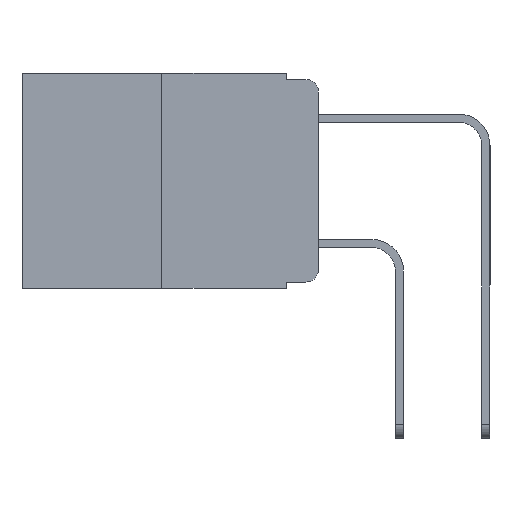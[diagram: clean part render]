
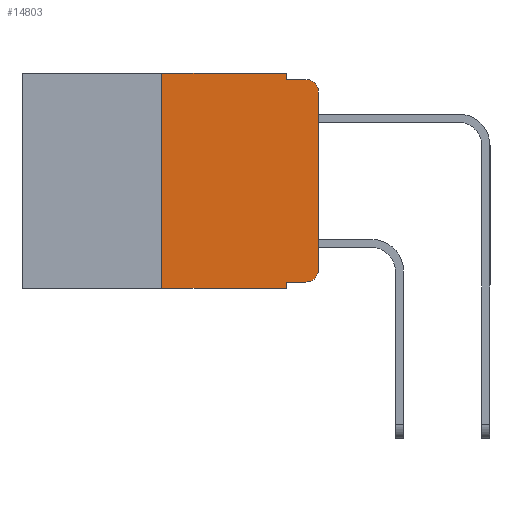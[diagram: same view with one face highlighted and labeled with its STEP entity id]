
A CAD part, left-side view. The second image highlights one B-rep face of the part: STEP entity #14803.
In plain terms, the highlighted planar face has unit normal (-1, 0, 0).
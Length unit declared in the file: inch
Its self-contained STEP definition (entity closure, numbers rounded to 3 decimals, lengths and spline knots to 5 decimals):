
#82 = VERTEX_POINT ( 'NONE', #9330 ) ;
#429 = VECTOR ( 'NONE', #21361, 39.37008 ) ;
#503 = AXIS2_PLACEMENT_3D ( 'NONE', #10269, #24353, #12307 ) ;
#767 = EDGE_CURVE ( 'NONE', #4249, #23061, #5872, .T. ) ;
#905 = VERTEX_POINT ( 'NONE', #11704 ) ;
#1455 = DIRECTION ( 'NONE',  ( 0., -1., 0. ) ) ;
#2556 = ORIENTED_EDGE ( 'NONE', *, *, #24773, .F. ) ;
#2732 = CARTESIAN_POINT ( 'NONE',  ( 0., 0., 0. ) ) ;
#3150 = DIRECTION ( 'NONE',  ( 0., -1., 0. ) ) ;
#3695 = CARTESIAN_POINT ( 'NONE',  ( 0., 0.051, -0.343 ) ) ;
#3861 = ORIENTED_EDGE ( 'NONE', *, *, #8584, .T. ) ;
#4249 = VERTEX_POINT ( 'NONE', #14105 ) ;
#4590 = DIRECTION ( 'NONE',  ( 0., 0., -1. ) ) ;
#4887 = EDGE_CURVE ( 'NONE', #23061, #9965, #10456, .T. ) ;
#5116 = AXIS2_PLACEMENT_3D ( 'NONE', #17857, #5764, #19891 ) ;
#5397 = LINE ( 'NONE', #20766, #15482 ) ;
#5639 = CARTESIAN_POINT ( 'NONE',  ( 0., 0.02, -0.333 ) ) ;
#5764 = DIRECTION ( 'NONE',  ( -1., 0., 0. ) ) ;
#5845 = LINE ( 'NONE', #2732, #21961 ) ;
#5872 = LINE ( 'NONE', #9257, #429 ) ;
#6551 = DIRECTION ( 'NONE',  ( 0., 0., -1. ) ) ;
#6782 = VERTEX_POINT ( 'NONE', #16998 ) ;
#7160 = EDGE_CURVE ( 'NONE', #16201, #9965, #9283, .T. ) ;
#8462 = EDGE_LOOP ( 'NONE', ( #9809, #11071, #23081, #13590, #24937, #16152, #12671, #2556, #3861, #25245 ) ) ;
#8567 = CARTESIAN_POINT ( 'NONE',  ( 0., 0.051, 0. ) ) ;
#8584 = EDGE_CURVE ( 'NONE', #82, #12564, #18343, .T. ) ;
#8742 = EDGE_CURVE ( 'NONE', #21947, #26122, #14508, .T. ) ;
#8759 = CARTESIAN_POINT ( 'NONE',  ( 0., 0., -0.03 ) ) ;
#9257 = CARTESIAN_POINT ( 'NONE',  ( 0., 0.051, 0. ) ) ;
#9283 = CIRCLE ( 'NONE', #503, 0.02 ) ;
#9330 = CARTESIAN_POINT ( 'NONE',  ( 0., 0.051, -0.333 ) ) ;
#9809 = ORIENTED_EDGE ( 'NONE', *, *, #25117, .T. ) ;
#9965 = VERTEX_POINT ( 'NONE', #13839 ) ;
#10269 = CARTESIAN_POINT ( 'NONE',  ( 0., 0.02, -0.03 ) ) ;
#10456 = LINE ( 'NONE', #20638, #20577 ) ;
#10733 = FACE_OUTER_BOUND ( 'NONE', #8462, .T. ) ;
#11071 = ORIENTED_EDGE ( 'NONE', *, *, #7160, .T. ) ;
#11704 = CARTESIAN_POINT ( 'NONE',  ( 0., 0.25, 0. ) ) ;
#12077 = DIRECTION ( 'NONE',  ( 0., -1., 0. ) ) ;
#12307 = DIRECTION ( 'NONE',  ( 0., 0., -1. ) ) ;
#12564 = VERTEX_POINT ( 'NONE', #5639 ) ;
#12624 = CARTESIAN_POINT ( 'NONE',  ( 0., 0.473, 0. ) ) ;
#12671 = ORIENTED_EDGE ( 'NONE', *, *, #8742, .T. ) ;
#13590 = ORIENTED_EDGE ( 'NONE', *, *, #767, .F. ) ;
#13704 = EDGE_CURVE ( 'NONE', #905, #4249, #25260, .T. ) ;
#13839 = CARTESIAN_POINT ( 'NONE',  ( 0., 0.02, -0.01 ) ) ;
#14105 = CARTESIAN_POINT ( 'NONE',  ( 0., 0.051, 0. ) ) ;
#14508 = LINE ( 'NONE', #16131, #19284 ) ;
#14679 = DIRECTION ( 'NONE',  ( 0., -1., 0. ) ) ;
#14803 = ADVANCED_FACE ( 'NONE', ( #10733 ), #18641, .F. ) ;
#14817 = DIRECTION ( 'NONE',  ( 0., 0., 1. ) ) ;
#14830 = EDGE_CURVE ( 'NONE', #21947, #905, #5397, .T. ) ;
#15216 = CARTESIAN_POINT ( 'NONE',  ( 0., 0.473, 0. ) ) ;
#15482 = VECTOR ( 'NONE', #22771, 39.37008 ) ;
#15890 = AXIS2_PLACEMENT_3D ( 'NONE', #12624, #16675, #4590 ) ;
#16131 = CARTESIAN_POINT ( 'NONE',  ( 0., 0.473, -0.343 ) ) ;
#16152 = ORIENTED_EDGE ( 'NONE', *, *, #14830, .F. ) ;
#16201 = VERTEX_POINT ( 'NONE', #8759 ) ;
#16675 = DIRECTION ( 'NONE',  ( 1., 0., 0. ) ) ;
#16998 = CARTESIAN_POINT ( 'NONE',  ( 0., 0., -0.313 ) ) ;
#17216 = EDGE_CURVE ( 'NONE', #12564, #6782, #17576, .T. ) ;
#17576 = CIRCLE ( 'NONE', #5116, 0.02 ) ;
#17857 = CARTESIAN_POINT ( 'NONE',  ( 0., 0.02, -0.313 ) ) ;
#18343 = LINE ( 'NONE', #25599, #18976 ) ;
#18641 = PLANE ( 'NONE',  #15890 ) ;
#18976 = VECTOR ( 'NONE', #1455, 39.37008 ) ;
#19284 = VECTOR ( 'NONE', #12077, 39.37008 ) ;
#19891 = DIRECTION ( 'NONE',  ( 0., 0., -1. ) ) ;
#20577 = VECTOR ( 'NONE', #14679, 39.37008 ) ;
#20638 = CARTESIAN_POINT ( 'NONE',  ( 0., 0.051, -0.01 ) ) ;
#20766 = CARTESIAN_POINT ( 'NONE',  ( 0., 0.25, 0. ) ) ;
#21361 = DIRECTION ( 'NONE',  ( 0., 0., -1. ) ) ;
#21947 = VERTEX_POINT ( 'NONE', #24531 ) ;
#21961 = VECTOR ( 'NONE', #14817, 39.37008 ) ;
#22771 = DIRECTION ( 'NONE',  ( 0., 0., 1. ) ) ;
#22857 = CARTESIAN_POINT ( 'NONE',  ( 0., 0.051, -0.01 ) ) ;
#23061 = VERTEX_POINT ( 'NONE', #22857 ) ;
#23081 = ORIENTED_EDGE ( 'NONE', *, *, #4887, .F. ) ;
#24353 = DIRECTION ( 'NONE',  ( -1., 0., 0. ) ) ;
#24531 = CARTESIAN_POINT ( 'NONE',  ( 0., 0.25, -0.343 ) ) ;
#24735 = LINE ( 'NONE', #8567, #25969 ) ;
#24773 = EDGE_CURVE ( 'NONE', #82, #26122, #24735, .T. ) ;
#24937 = ORIENTED_EDGE ( 'NONE', *, *, #13704, .F. ) ;
#25117 = EDGE_CURVE ( 'NONE', #6782, #16201, #5845, .T. ) ;
#25245 = ORIENTED_EDGE ( 'NONE', *, *, #17216, .T. ) ;
#25260 = LINE ( 'NONE', #15216, #25896 ) ;
#25599 = CARTESIAN_POINT ( 'NONE',  ( 0., 0.051, -0.333 ) ) ;
#25896 = VECTOR ( 'NONE', #3150, 39.37008 ) ;
#25969 = VECTOR ( 'NONE', #6551, 39.37008 ) ;
#26122 = VERTEX_POINT ( 'NONE', #3695 ) ;
